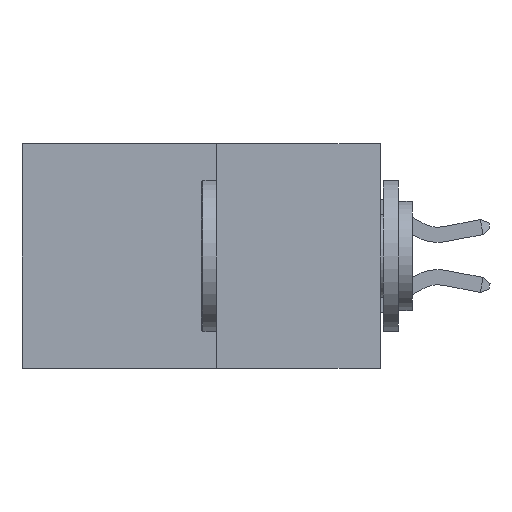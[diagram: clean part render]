
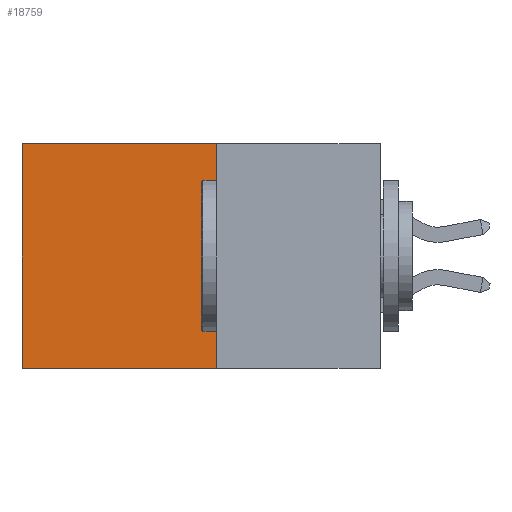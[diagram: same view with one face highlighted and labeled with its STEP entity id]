
A CAD part, left-side view. The second image highlights one B-rep face of the part: STEP entity #18759.
In plain terms, the highlighted planar face has unit normal (-1, 0, 0).
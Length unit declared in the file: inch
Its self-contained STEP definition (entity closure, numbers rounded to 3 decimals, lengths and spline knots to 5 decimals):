
#722 = CARTESIAN_POINT ( 'NONE',  ( 0.277, 0.27, -0.37 ) ) ;
#819 = VERTEX_POINT ( 'NONE', #12162 ) ;
#3130 = VECTOR ( 'NONE', #10360, 39.37008 ) ;
#4795 = DIRECTION ( 'NONE',  ( 0., 0., -1. ) ) ;
#5554 = CARTESIAN_POINT ( 'NONE',  ( 0.277, 0.27, -0.37 ) ) ;
#6531 = ORIENTED_EDGE ( 'NONE', *, *, #11083, .F. ) ;
#7011 = VERTEX_POINT ( 'NONE', #5554 ) ;
#7421 = DIRECTION ( 'NONE',  ( 0., 0., -1. ) ) ;
#7760 = EDGE_CURVE ( 'NONE', #819, #22780, #16254, .T. ) ;
#8128 = CARTESIAN_POINT ( 'NONE',  ( 0.277, 0.27, 0. ) ) ;
#8169 = CARTESIAN_POINT ( 'NONE',  ( 0.277, 0.27, -0.37 ) ) ;
#8360 = LINE ( 'NONE', #8128, #3130 ) ;
#9205 = CARTESIAN_POINT ( 'NONE',  ( 0.277, 0.27, -0.37 ) ) ;
#9369 = VECTOR ( 'NONE', #16949, 39.37008 ) ;
#10192 = FACE_OUTER_BOUND ( 'NONE', #12002, .T. ) ;
#10360 = DIRECTION ( 'NONE',  ( 0., 1., 0. ) ) ;
#10506 = VECTOR ( 'NONE', #4795, 39.37008 ) ;
#11083 = EDGE_CURVE ( 'NONE', #27288, #7011, #14244, .T. ) ;
#12002 = EDGE_LOOP ( 'NONE', ( #23846, #26595, #6531, #27287 ) ) ;
#12162 = CARTESIAN_POINT ( 'NONE',  ( 0.277, 0.59, 0. ) ) ;
#13555 = VECTOR ( 'NONE', #22213, 39.37008 ) ;
#14244 = LINE ( 'NONE', #9205, #13555 ) ;
#15177 = LINE ( 'NONE', #8169, #9369 ) ;
#16111 = PLANE ( 'NONE',  #23922 ) ;
#16254 = LINE ( 'NONE', #27326, #10506 ) ;
#16949 = DIRECTION ( 'NONE',  ( 0., 1., 0. ) ) ;
#18759 = ADVANCED_FACE ( 'NONE', ( #10192 ), #16111, .F. ) ;
#20394 = EDGE_CURVE ( 'NONE', #27288, #819, #8360, .T. ) ;
#20480 = DIRECTION ( 'NONE',  ( 1., 0., 0. ) ) ;
#20862 = CARTESIAN_POINT ( 'NONE',  ( 0.277, 0.59, -0.37 ) ) ;
#22213 = DIRECTION ( 'NONE',  ( 0., 0., -1. ) ) ;
#22780 = VERTEX_POINT ( 'NONE', #20862 ) ;
#23846 = ORIENTED_EDGE ( 'NONE', *, *, #7760, .T. ) ;
#23922 = AXIS2_PLACEMENT_3D ( 'NONE', #722, #20480, #7421 ) ;
#26215 = EDGE_CURVE ( 'NONE', #7011, #22780, #15177, .T. ) ;
#26595 = ORIENTED_EDGE ( 'NONE', *, *, #26215, .F. ) ;
#26815 = CARTESIAN_POINT ( 'NONE',  ( 0.277, 0.27, 0. ) ) ;
#27287 = ORIENTED_EDGE ( 'NONE', *, *, #20394, .T. ) ;
#27288 = VERTEX_POINT ( 'NONE', #26815 ) ;
#27326 = CARTESIAN_POINT ( 'NONE',  ( 0.277, 0.59, -0.37 ) ) ;
